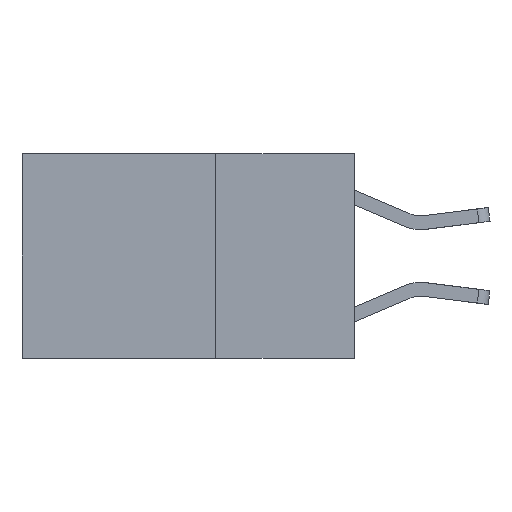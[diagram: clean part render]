
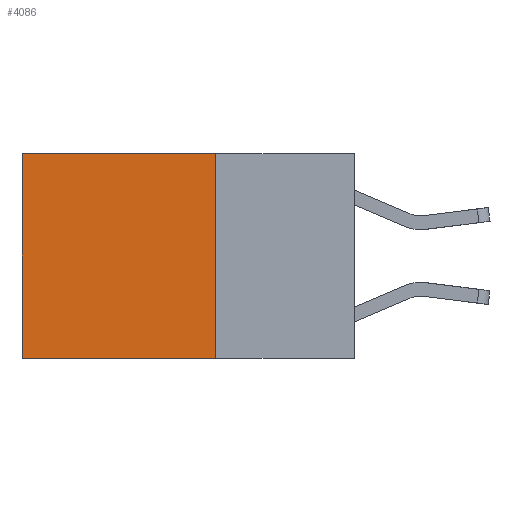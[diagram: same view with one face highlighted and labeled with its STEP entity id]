
A CAD part, left-side view. The second image highlights one B-rep face of the part: STEP entity #4086.
In plain terms, the highlighted planar face has unit normal (-1, 0, 0).
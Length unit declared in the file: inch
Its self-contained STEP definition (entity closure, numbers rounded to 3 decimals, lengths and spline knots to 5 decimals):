
#62 = DIRECTION ( 'NONE',  ( 0., 0., -1. ) ) ;
#323 = DIRECTION ( 'NONE',  ( 0., 0., -1. ) ) ;
#603 = VERTEX_POINT ( 'NONE', #4532 ) ;
#889 = FACE_OUTER_BOUND ( 'NONE', #4226, .T. ) ;
#1188 = LINE ( 'NONE', #3591, #4718 ) ;
#1305 = LINE ( 'NONE', #4997, #4261 ) ;
#1329 = EDGE_CURVE ( 'NONE', #1641, #3404, #1305, .T. ) ;
#1374 = EDGE_CURVE ( 'NONE', #1641, #7223, #1188, .T. ) ;
#1483 = CARTESIAN_POINT ( 'NONE',  ( 0.2625, 0.25, 0. ) ) ;
#1641 = VERTEX_POINT ( 'NONE', #3445 ) ;
#1861 = AXIS2_PLACEMENT_3D ( 'NONE', #1483, #2196, #62 ) ;
#2150 = DIRECTION ( 'NONE',  ( 0., 1., 0. ) ) ;
#2196 = DIRECTION ( 'NONE',  ( 1., 0., 0. ) ) ;
#2866 = ORIENTED_EDGE ( 'NONE', *, *, #1329, .F. ) ;
#3073 = LINE ( 'NONE', #4872, #6579 ) ;
#3404 = VERTEX_POINT ( 'NONE', #7434 ) ;
#3445 = CARTESIAN_POINT ( 'NONE',  ( 0.2625, 0.25, 0. ) ) ;
#3591 = CARTESIAN_POINT ( 'NONE',  ( 0.2625, 0.25, 0. ) ) ;
#3758 = ORIENTED_EDGE ( 'NONE', *, *, #5523, .F. ) ;
#3887 = ORIENTED_EDGE ( 'NONE', *, *, #1374, .T. ) ;
#4086 = ADVANCED_FACE ( 'NONE', ( #889 ), #5623, .F. ) ;
#4226 = EDGE_LOOP ( 'NONE', ( #7475, #3758, #2866, #3887 ) ) ;
#4261 = VECTOR ( 'NONE', #7059, 39.37008 ) ;
#4427 = LINE ( 'NONE', #4498, #5090 ) ;
#4498 = CARTESIAN_POINT ( 'NONE',  ( 0.2625, 0.6, 0. ) ) ;
#4532 = CARTESIAN_POINT ( 'NONE',  ( 0.2625, 0.6, -0.37 ) ) ;
#4718 = VECTOR ( 'NONE', #8519, 39.37008 ) ;
#4872 = CARTESIAN_POINT ( 'NONE',  ( 0.2625, 0.25, -0.37 ) ) ;
#4997 = CARTESIAN_POINT ( 'NONE',  ( 0.2625, 0.25, 0. ) ) ;
#5090 = VECTOR ( 'NONE', #323, 39.37008 ) ;
#5523 = EDGE_CURVE ( 'NONE', #3404, #603, #3073, .T. ) ;
#5623 = PLANE ( 'NONE',  #1861 ) ;
#6579 = VECTOR ( 'NONE', #2150, 39.37008 ) ;
#7059 = DIRECTION ( 'NONE',  ( 0., 0., -1. ) ) ;
#7223 = VERTEX_POINT ( 'NONE', #7448 ) ;
#7434 = CARTESIAN_POINT ( 'NONE',  ( 0.2625, 0.25, -0.37 ) ) ;
#7448 = CARTESIAN_POINT ( 'NONE',  ( 0.2625, 0.6, 0. ) ) ;
#7475 = ORIENTED_EDGE ( 'NONE', *, *, #8506, .T. ) ;
#8506 = EDGE_CURVE ( 'NONE', #7223, #603, #4427, .T. ) ;
#8519 = DIRECTION ( 'NONE',  ( 0., 1., 0. ) ) ;
